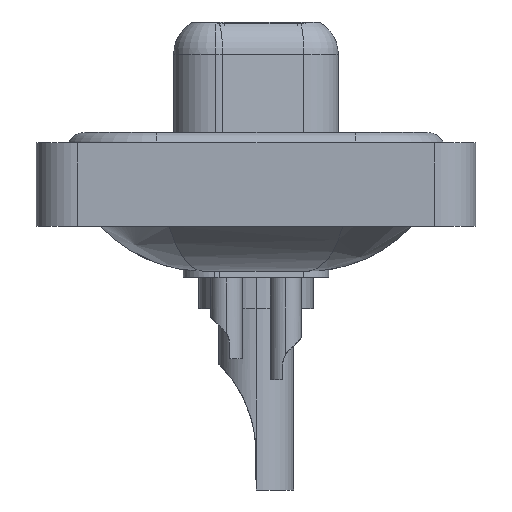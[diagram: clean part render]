
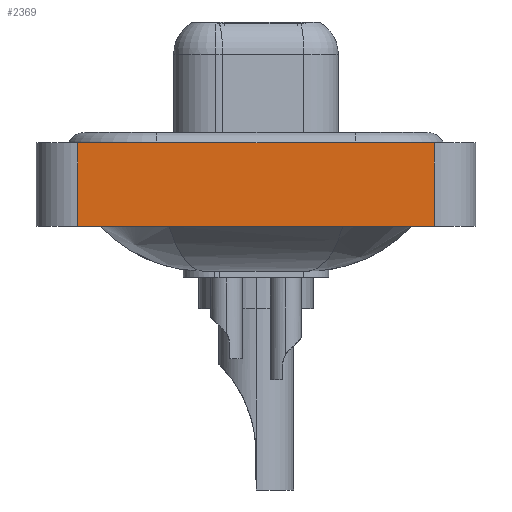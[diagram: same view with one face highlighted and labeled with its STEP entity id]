
A CAD part, left-side view. The second image highlights one B-rep face of the part: STEP entity #2369.
In plain terms, the highlighted planar face has unit normal (-1, 0, 0).
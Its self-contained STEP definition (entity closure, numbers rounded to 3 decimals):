
#976 = EDGE_CURVE ( 'NONE', #9672, #6214, #11964, .T. ) ;
#1324 = CARTESIAN_POINT ( 'NONE',  ( -7.3, -8.55, -3.6 ) ) ;
#2369 = ADVANCED_FACE ( 'NONE', ( #3785 ), #5284, .T. ) ;
#2650 = CARTESIAN_POINT ( 'NONE',  ( -7.3, -8.55, -3.6 ) ) ;
#2668 = EDGE_LOOP ( 'NONE', ( #10460, #9509, #7073, #11239 ) ) ;
#3045 = CARTESIAN_POINT ( 'NONE',  ( -7.3, 8.55, -3.6 ) ) ;
#3785 = FACE_OUTER_BOUND ( 'NONE', #2668, .T. ) ;
#4277 = VECTOR ( 'NONE', #14693, 1000. ) ;
#4429 = LINE ( 'NONE', #17903, #4277 ) ;
#5284 = PLANE ( 'NONE',  #12421 ) ;
#6214 = VERTEX_POINT ( 'NONE', #14529 ) ;
#6790 = DIRECTION ( 'NONE',  ( -1., 0., 0. ) ) ;
#7073 = ORIENTED_EDGE ( 'NONE', *, *, #13769, .F. ) ;
#9509 = ORIENTED_EDGE ( 'NONE', *, *, #11774, .F. ) ;
#9672 = VERTEX_POINT ( 'NONE', #2650 ) ;
#10027 = CARTESIAN_POINT ( 'NONE',  ( -7.3, 8.55, -3.6 ) ) ;
#10043 = DIRECTION ( 'NONE',  ( 0., 0., 1. ) ) ;
#10368 = VECTOR ( 'NONE', #15380, 1000. ) ;
#10460 = ORIENTED_EDGE ( 'NONE', *, *, #976, .T. ) ;
#11239 = ORIENTED_EDGE ( 'NONE', *, *, #13128, .T. ) ;
#11664 = CARTESIAN_POINT ( 'NONE',  ( -7.3, 8.55, 0.4 ) ) ;
#11774 = EDGE_CURVE ( 'NONE', #13618, #6214, #4429, .T. ) ;
#11964 = LINE ( 'NONE', #18959, #20048 ) ;
#12421 = AXIS2_PLACEMENT_3D ( 'NONE', #17475, #6790, #13823 ) ;
#12715 = DIRECTION ( 'NONE',  ( 0., 0., 1. ) ) ;
#13128 = EDGE_CURVE ( 'NONE', #21854, #9672, #21901, .T. ) ;
#13618 = VERTEX_POINT ( 'NONE', #11664 ) ;
#13769 = EDGE_CURVE ( 'NONE', #21854, #13618, #22452, .T. ) ;
#13823 = DIRECTION ( 'NONE',  ( 0., 0., 1. ) ) ;
#14529 = CARTESIAN_POINT ( 'NONE',  ( -7.3, -8.55, 0.4 ) ) ;
#14693 = DIRECTION ( 'NONE',  ( 0., -1., 0. ) ) ;
#15380 = DIRECTION ( 'NONE',  ( 0., -1., 0. ) ) ;
#17475 = CARTESIAN_POINT ( 'NONE',  ( -7.3, -8.55, -3.6 ) ) ;
#17903 = CARTESIAN_POINT ( 'NONE',  ( -7.3, -8.55, 0.4 ) ) ;
#18959 = CARTESIAN_POINT ( 'NONE',  ( -7.3, -8.55, -3.6 ) ) ;
#20048 = VECTOR ( 'NONE', #12715, 1000. ) ;
#21027 = VECTOR ( 'NONE', #10043, 1000. ) ;
#21854 = VERTEX_POINT ( 'NONE', #10027 ) ;
#21901 = LINE ( 'NONE', #1324, #10368 ) ;
#22452 = LINE ( 'NONE', #3045, #21027 ) ;
